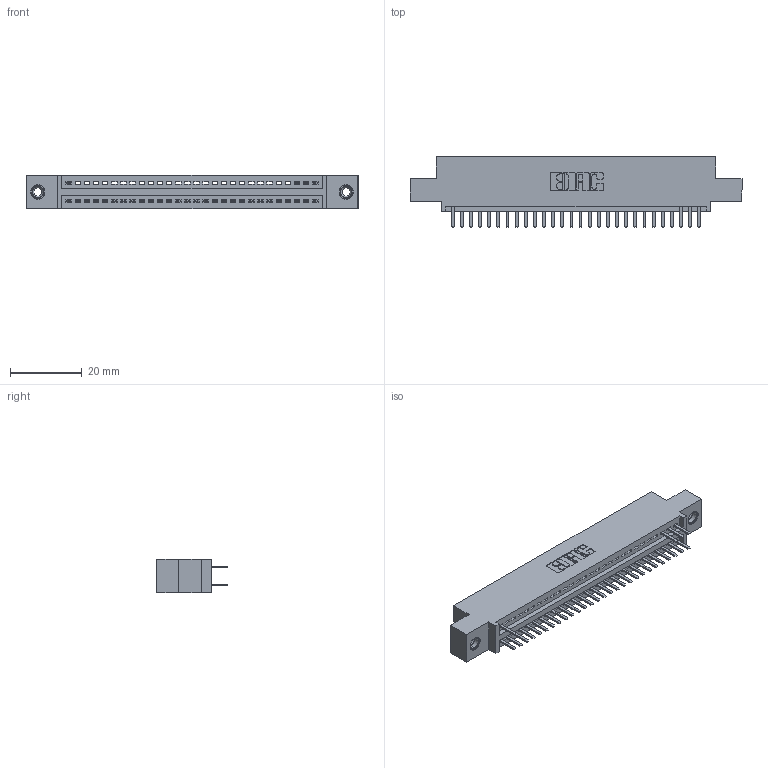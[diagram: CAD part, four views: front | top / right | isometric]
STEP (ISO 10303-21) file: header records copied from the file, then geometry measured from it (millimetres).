
FILE_DESCRIPTION (( 'STEP AP203' ), '1' );
FILE_NAME ('345-056-520-508.STEP', '2018-09-24T07:07:57', ( '' ), ( '' ), 'SwSTEP 2.0', 'SolidWorks 2016', '' );
FILE_SCHEMA (( 'CONFIG_CONTROL_DESIGN' ));
Length unit declared in the file: inch
Products named in the file (4): 345-292-001_345-293-120; 345-250-001_345-250-003-102; 345-056-520-508; 345 Part_0.110 Offset - 0.156 Dia-TI
Assembly tree (35 placements, depth 2):
  345-056-520-508
    345 Part_0.110 Offset - 0.156 Dia-TI
    345-292-001_345-293-120  x32
    345-250-001_345-250-003-102  x2
Bounding box: 92.33 x 19.68 x 9.4 mm (x, y, z)
Volume: 8528.7 mm3; surface area: 11186.7 mm2
Topology: 35 solids, 35 shells, 2110 faces, 6161 edges, 4014 vertices
Faces by surface type: plane 1404, cylinder 690, cone 12, torus 4
Entity records: 24518 total; most frequent: CARTESIAN_POINT 4223, ORIENTED_EDGE 4162, DIRECTION 3727, EDGE_CURVE 2081, VECTOR 1813, LINE 1813, VERTEX_POINT 1380, AXIS2_PLACEMENT_3D 957
